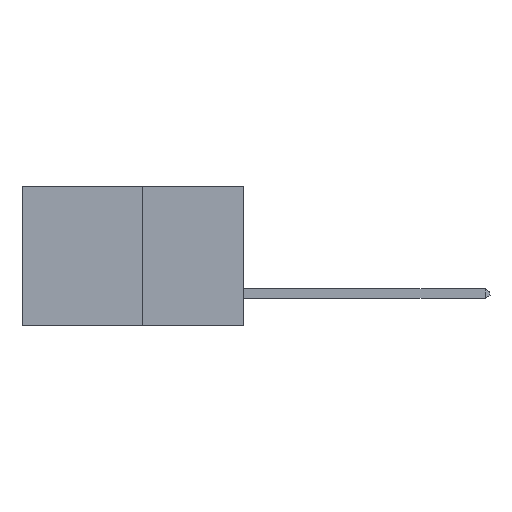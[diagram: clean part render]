
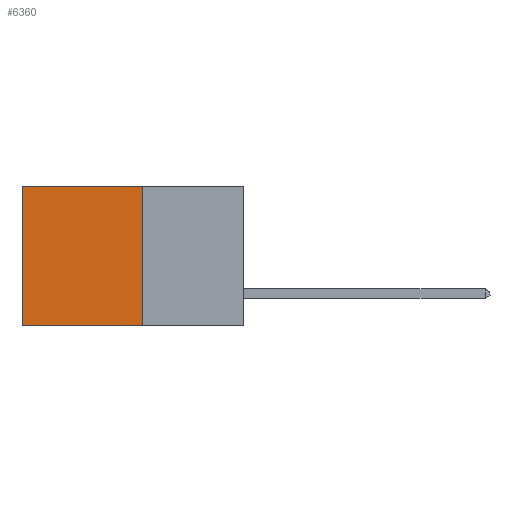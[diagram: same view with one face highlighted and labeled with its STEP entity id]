
A CAD part, left-side view. The second image highlights one B-rep face of the part: STEP entity #6360.
In plain terms, the highlighted planar face has unit normal (-1, 0, 0).
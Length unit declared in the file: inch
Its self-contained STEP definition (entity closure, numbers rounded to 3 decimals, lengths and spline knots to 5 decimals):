
#215 = DIRECTION ( 'NONE',  ( 0., 0., -1. ) ) ;
#841 = LINE ( 'NONE', #3346, #4891 ) ;
#1336 = VECTOR ( 'NONE', #215, 39.37008 ) ;
#1599 = VERTEX_POINT ( 'NONE', #6839 ) ;
#1626 = CARTESIAN_POINT ( 'NONE',  ( 0.277, 0.27, -0.37 ) ) ;
#2034 = EDGE_CURVE ( 'NONE', #6873, #1599, #5307, .T. ) ;
#2324 = DIRECTION ( 'NONE',  ( 0., 1., 0. ) ) ;
#2796 = DIRECTION ( 'NONE',  ( 0., 1., 0. ) ) ;
#2989 = VECTOR ( 'NONE', #4457, 39.37008 ) ;
#3119 = AXIS2_PLACEMENT_3D ( 'NONE', #5219, #4681, #4331 ) ;
#3346 = CARTESIAN_POINT ( 'NONE',  ( 0.277, 0.27, -0.37 ) ) ;
#3698 = PLANE ( 'NONE',  #3119 ) ;
#4331 = DIRECTION ( 'NONE',  ( 0., 0., -1. ) ) ;
#4457 = DIRECTION ( 'NONE',  ( 0., 0., -1. ) ) ;
#4681 = DIRECTION ( 'NONE',  ( 1., 0., 0. ) ) ;
#4891 = VECTOR ( 'NONE', #2796, 39.37008 ) ;
#4922 = CARTESIAN_POINT ( 'NONE',  ( 0.277, 0.59, 0. ) ) ;
#4977 = ORIENTED_EDGE ( 'NONE', *, *, #9232, .T. ) ;
#5185 = EDGE_LOOP ( 'NONE', ( #6141, #8512, #5630, #4977 ) ) ;
#5219 = CARTESIAN_POINT ( 'NONE',  ( 0.277, 0.27, -0.37 ) ) ;
#5307 = LINE ( 'NONE', #7410, #2989 ) ;
#5630 = ORIENTED_EDGE ( 'NONE', *, *, #6687, .F. ) ;
#5992 = CARTESIAN_POINT ( 'NONE',  ( 0.277, 0.27, 0. ) ) ;
#6141 = ORIENTED_EDGE ( 'NONE', *, *, #2034, .T. ) ;
#6263 = EDGE_CURVE ( 'NONE', #9317, #1599, #841, .T. ) ;
#6360 = ADVANCED_FACE ( 'NONE', ( #7779 ), #3698, .F. ) ;
#6687 = EDGE_CURVE ( 'NONE', #7024, #9317, #9044, .T. ) ;
#6839 = CARTESIAN_POINT ( 'NONE',  ( 0.277, 0.59, -0.37 ) ) ;
#6873 = VERTEX_POINT ( 'NONE', #4922 ) ;
#7024 = VERTEX_POINT ( 'NONE', #7229 ) ;
#7229 = CARTESIAN_POINT ( 'NONE',  ( 0.277, 0.27, 0. ) ) ;
#7410 = CARTESIAN_POINT ( 'NONE',  ( 0.277, 0.59, -0.37 ) ) ;
#7626 = VECTOR ( 'NONE', #2324, 39.37008 ) ;
#7779 = FACE_OUTER_BOUND ( 'NONE', #5185, .T. ) ;
#8264 = CARTESIAN_POINT ( 'NONE',  ( 0.277, 0.27, -0.37 ) ) ;
#8512 = ORIENTED_EDGE ( 'NONE', *, *, #6263, .F. ) ;
#9044 = LINE ( 'NONE', #8264, #1336 ) ;
#9232 = EDGE_CURVE ( 'NONE', #7024, #6873, #9409, .T. ) ;
#9317 = VERTEX_POINT ( 'NONE', #1626 ) ;
#9409 = LINE ( 'NONE', #5992, #7626 ) ;
